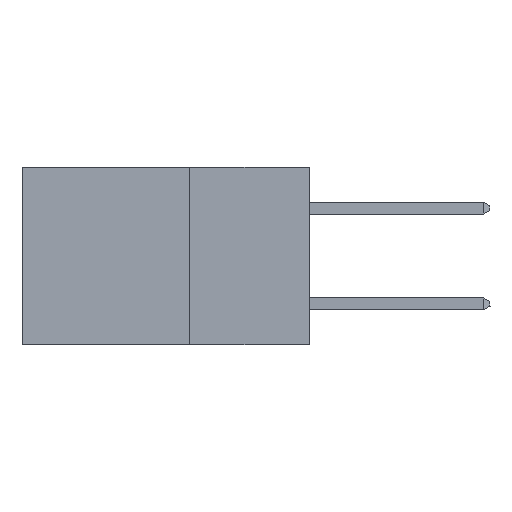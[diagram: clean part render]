
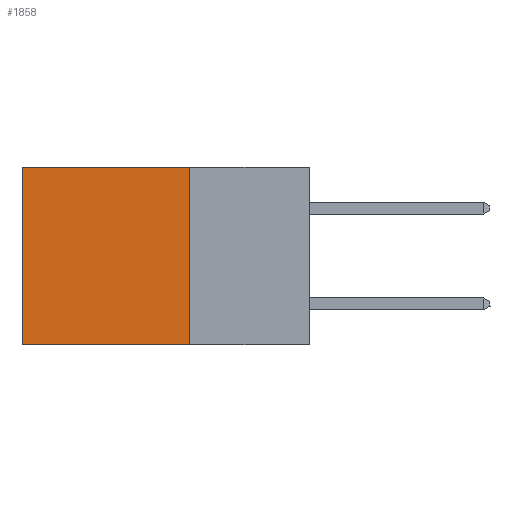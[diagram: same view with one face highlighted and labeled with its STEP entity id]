
A CAD part, left-side view. The second image highlights one B-rep face of the part: STEP entity #1858.
In plain terms, the highlighted planar face has unit normal (-1, 0, 0).
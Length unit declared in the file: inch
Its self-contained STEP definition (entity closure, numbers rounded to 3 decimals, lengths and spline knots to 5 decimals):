
#895 = CARTESIAN_POINT ( 'NONE',  ( 0.2875, 0.25, -0.37 ) ) ;
#1307 = DIRECTION ( 'NONE',  ( 0., 1., 0. ) ) ;
#1858 = ADVANCED_FACE ( 'NONE', ( #3350 ), #2511, .F. ) ;
#2169 = CARTESIAN_POINT ( 'NONE',  ( 0.2875, 0.6, -0.37 ) ) ;
#2334 = VECTOR ( 'NONE', #9932, 39.37008 ) ;
#2485 = VECTOR ( 'NONE', #1307, 39.37008 ) ;
#2511 = PLANE ( 'NONE',  #19597 ) ;
#3350 = FACE_OUTER_BOUND ( 'NONE', #24486, .T. ) ;
#3736 = CARTESIAN_POINT ( 'NONE',  ( 0.2875, 0.25, -0.37 ) ) ;
#4521 = DIRECTION ( 'NONE',  ( 0., 0., -1. ) ) ;
#4571 = EDGE_CURVE ( 'NONE', #13186, #20954, #14716, .T. ) ;
#5611 = DIRECTION ( 'NONE',  ( 0., 0., -1. ) ) ;
#5867 = CARTESIAN_POINT ( 'NONE',  ( 0.2875, 0.6, 0. ) ) ;
#7049 = LINE ( 'NONE', #5867, #7973 ) ;
#7607 = CARTESIAN_POINT ( 'NONE',  ( 0.2875, 0.25, 0. ) ) ;
#7687 = VERTEX_POINT ( 'NONE', #20157 ) ;
#7973 = VECTOR ( 'NONE', #5611, 39.37008 ) ;
#8402 = DIRECTION ( 'NONE',  ( 1., 0., 0. ) ) ;
#9932 = DIRECTION ( 'NONE',  ( 0., 0., -1. ) ) ;
#10606 = ORIENTED_EDGE ( 'NONE', *, *, #16132, .F. ) ;
#11969 = DIRECTION ( 'NONE',  ( 0., 1., 0. ) ) ;
#12557 = CARTESIAN_POINT ( 'NONE',  ( 0.2875, 0.25, 0. ) ) ;
#12653 = VERTEX_POINT ( 'NONE', #16758 ) ;
#12677 = ORIENTED_EDGE ( 'NONE', *, *, #13308, .T. ) ;
#13186 = VERTEX_POINT ( 'NONE', #895 ) ;
#13308 = EDGE_CURVE ( 'NONE', #12653, #7687, #14320, .T. ) ;
#14320 = LINE ( 'NONE', #17173, #2485 ) ;
#14716 = LINE ( 'NONE', #3736, #24098 ) ;
#16132 = EDGE_CURVE ( 'NONE', #12653, #13186, #21038, .T. ) ;
#16601 = ORIENTED_EDGE ( 'NONE', *, *, #4571, .F. ) ;
#16758 = CARTESIAN_POINT ( 'NONE',  ( 0.2875, 0.25, 0. ) ) ;
#17151 = EDGE_CURVE ( 'NONE', #7687, #20954, #7049, .T. ) ;
#17173 = CARTESIAN_POINT ( 'NONE',  ( 0.2875, 0.25, 0. ) ) ;
#19587 = ORIENTED_EDGE ( 'NONE', *, *, #17151, .T. ) ;
#19597 = AXIS2_PLACEMENT_3D ( 'NONE', #12557, #8402, #4521 ) ;
#20157 = CARTESIAN_POINT ( 'NONE',  ( 0.2875, 0.6, 0. ) ) ;
#20954 = VERTEX_POINT ( 'NONE', #2169 ) ;
#21038 = LINE ( 'NONE', #7607, #2334 ) ;
#24098 = VECTOR ( 'NONE', #11969, 39.37008 ) ;
#24486 = EDGE_LOOP ( 'NONE', ( #19587, #16601, #10606, #12677 ) ) ;
